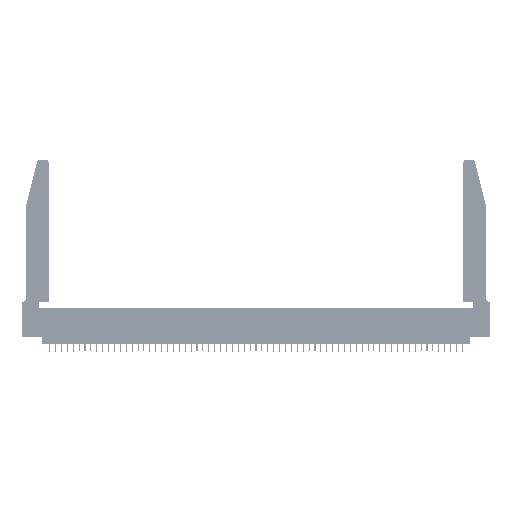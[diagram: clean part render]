
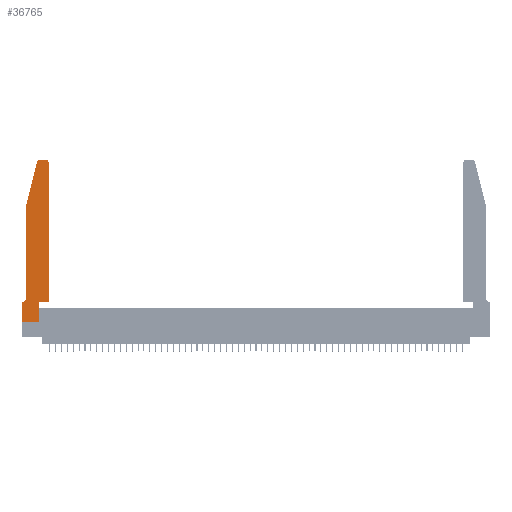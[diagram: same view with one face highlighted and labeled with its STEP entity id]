
A CAD part, top view. The second image highlights one B-rep face of the part: STEP entity #36765.
In plain terms, the highlighted planar face has unit normal (0, 0, 1).
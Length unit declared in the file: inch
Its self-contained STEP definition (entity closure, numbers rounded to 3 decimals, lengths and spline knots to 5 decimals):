
#133 = DIRECTION ( 'NONE',  ( -0.239, -0.971, 0. ) ) ;
#242 = VERTEX_POINT ( 'NONE', #3812 ) ;
#256 = CARTESIAN_POINT ( 'NONE',  ( 0.4205, 2.72, 0.37 ) ) ;
#416 = CARTESIAN_POINT ( 'NONE',  ( 0.0055, 0.42, 0.37 ) ) ;
#636 = DIRECTION ( 'NONE',  ( 0., 1., 0. ) ) ;
#1036 = CARTESIAN_POINT ( 'NONE',  ( 0.4505, 2.72, 0.37 ) ) ;
#1642 = VERTEX_POINT ( 'NONE', #56028 ) ;
#1770 = DIRECTION ( 'NONE',  ( 0., -1., 0. ) ) ;
#2079 = CARTESIAN_POINT ( 'NONE',  ( 0.2865, 0.35, 0.37 ) ) ;
#3624 = DIRECTION ( 'NONE',  ( 0., 0., -1. ) ) ;
#3812 = CARTESIAN_POINT ( 'NONE',  ( 0.0755, 0.42, 0.37 ) ) ;
#4233 = LINE ( 'NONE', #22372, #9941 ) ;
#4874 = EDGE_CURVE ( 'NONE', #10072, #18969, #46197, .T. ) ;
#4954 = LINE ( 'NONE', #40005, #13752 ) ;
#6051 = CARTESIAN_POINT ( 'NONE',  ( 0., 0.35, 0.37 ) ) ;
#8897 = DIRECTION ( 'NONE',  ( 1., 0., 0. ) ) ;
#8932 = EDGE_CURVE ( 'NONE', #41406, #28362, #38608, .T. ) ;
#9508 = CARTESIAN_POINT ( 'NONE',  ( 0.4205, 2.75, 0.37 ) ) ;
#9941 = VECTOR ( 'NONE', #21232, 39.37008 ) ;
#10072 = VERTEX_POINT ( 'NONE', #12974 ) ;
#10731 = VERTEX_POINT ( 'NONE', #45326 ) ;
#11606 = AXIS2_PLACEMENT_3D ( 'NONE', #15810, #56306, #50840 ) ;
#11866 = VERTEX_POINT ( 'NONE', #34751 ) ;
#12131 = AXIS2_PLACEMENT_3D ( 'NONE', #416, #3624, #21180 ) ;
#12811 = CARTESIAN_POINT ( 'NONE',  ( 0.0755, 2., 0.37 ) ) ;
#12974 = CARTESIAN_POINT ( 'NONE',  ( 0.284, 2.75, 0.37 ) ) ;
#13752 = VECTOR ( 'NONE', #636, 39.37008 ) ;
#14087 = EDGE_CURVE ( 'NONE', #1642, #19482, #4233, .T. ) ;
#14228 = LINE ( 'NONE', #48415, #37385 ) ;
#14549 = DIRECTION ( 'NONE',  ( 1., 0., 0. ) ) ;
#14752 = DIRECTION ( 'NONE',  ( 1., 0., 0. ) ) ;
#15810 = CARTESIAN_POINT ( 'NONE',  ( 0., 0.35, 0.37 ) ) ;
#15843 = EDGE_CURVE ( 'NONE', #18969, #26287, #36752, .T. ) ;
#15962 = ORIENTED_EDGE ( 'NONE', *, *, #15843, .T. ) ;
#17967 = DIRECTION ( 'NONE',  ( 1., 0., 0. ) ) ;
#18969 = VERTEX_POINT ( 'NONE', #40015 ) ;
#19440 = VERTEX_POINT ( 'NONE', #9508 ) ;
#19482 = VERTEX_POINT ( 'NONE', #6051 ) ;
#19561 = FACE_OUTER_BOUND ( 'NONE', #33764, .T. ) ;
#21128 = DIRECTION ( 'NONE',  ( 0., 1., 0. ) ) ;
#21180 = DIRECTION ( 'NONE',  ( -1., 0., 0. ) ) ;
#21232 = DIRECTION ( 'NONE',  ( -1., 0., 0. ) ) ;
#21454 = AXIS2_PLACEMENT_3D ( 'NONE', #40386, #35789, #14549 ) ;
#21631 = VERTEX_POINT ( 'NONE', #1036 ) ;
#22372 = CARTESIAN_POINT ( 'NONE',  ( 0.0755, 0.35, 0.37 ) ) ;
#23289 = EDGE_CURVE ( 'NONE', #11866, #41406, #14228, .T. ) ;
#23376 = VECTOR ( 'NONE', #28044, 39.37008 ) ;
#23929 = LINE ( 'NONE', #33097, #39742 ) ;
#25244 = EDGE_CURVE ( 'NONE', #28362, #10731, #36829, .T. ) ;
#26287 = VERTEX_POINT ( 'NONE', #52406 ) ;
#27281 = DIRECTION ( 'NONE',  ( 0., 0., 1. ) ) ;
#27922 = ORIENTED_EDGE ( 'NONE', *, *, #47736, .T. ) ;
#28044 = DIRECTION ( 'NONE',  ( -1., 0., 0. ) ) ;
#28362 = VERTEX_POINT ( 'NONE', #2079 ) ;
#29214 = ORIENTED_EDGE ( 'NONE', *, *, #42809, .T. ) ;
#30078 = ORIENTED_EDGE ( 'NONE', *, *, #39623, .T. ) ;
#30539 = EDGE_CURVE ( 'NONE', #242, #1642, #53443, .T. ) ;
#30883 = ORIENTED_EDGE ( 'NONE', *, *, #32994, .T. ) ;
#31133 = CARTESIAN_POINT ( 'NONE',  ( 0., 0., 0.37 ) ) ;
#32994 = EDGE_CURVE ( 'NONE', #26287, #242, #23929, .T. ) ;
#33097 = CARTESIAN_POINT ( 'NONE',  ( 0.0755, 2., 0.37 ) ) ;
#33535 = VECTOR ( 'NONE', #21128, 39.37008 ) ;
#33764 = EDGE_LOOP ( 'NONE', ( #27922, #39253, #15962, #30883, #53707, #35197, #30078, #39022, #38485, #50624, #29214, #34914 ) ) ;
#33943 = VECTOR ( 'NONE', #133, 39.37008 ) ;
#34751 = CARTESIAN_POINT ( 'NONE',  ( 0., 0., 0.37 ) ) ;
#34914 = ORIENTED_EDGE ( 'NONE', *, *, #43722, .T. ) ;
#35197 = ORIENTED_EDGE ( 'NONE', *, *, #14087, .T. ) ;
#35789 = DIRECTION ( 'NONE',  ( 0., 0., 1. ) ) ;
#36752 = LINE ( 'NONE', #12811, #33943 ) ;
#36765 = ADVANCED_FACE ( 'NONE', ( #19561 ), #42214, .T. ) ;
#36829 = LINE ( 'NONE', #37955, #45639 ) ;
#37385 = VECTOR ( 'NONE', #17967, 39.37008 ) ;
#37955 = CARTESIAN_POINT ( 'NONE',  ( 0.4505, 0.35, 0.37 ) ) ;
#38485 = ORIENTED_EDGE ( 'NONE', *, *, #8932, .T. ) ;
#38608 = LINE ( 'NONE', #46959, #33535 ) ;
#39022 = ORIENTED_EDGE ( 'NONE', *, *, #23289, .T. ) ;
#39253 = ORIENTED_EDGE ( 'NONE', *, *, #4874, .T. ) ;
#39520 = AXIS2_PLACEMENT_3D ( 'NONE', #256, #27281, #8897 ) ;
#39623 = EDGE_CURVE ( 'NONE', #19482, #11866, #39985, .T. ) ;
#39742 = VECTOR ( 'NONE', #50316, 39.37008 ) ;
#39985 = LINE ( 'NONE', #31133, #49295 ) ;
#40005 = CARTESIAN_POINT ( 'NONE',  ( 0.4505, 0.35, 0.37 ) ) ;
#40015 = CARTESIAN_POINT ( 'NONE',  ( 0.25487, 2.72718, 0.37 ) ) ;
#40386 = CARTESIAN_POINT ( 'NONE',  ( 0.284, 2.72, 0.37 ) ) ;
#41406 = VERTEX_POINT ( 'NONE', #54318 ) ;
#41799 = CARTESIAN_POINT ( 'NONE',  ( 0.2605, 2.75, 0.37 ) ) ;
#42214 = PLANE ( 'NONE',  #11606 ) ;
#42809 = EDGE_CURVE ( 'NONE', #10731, #21631, #4954, .T. ) ;
#43722 = EDGE_CURVE ( 'NONE', #21631, #19440, #49629, .T. ) ;
#45326 = CARTESIAN_POINT ( 'NONE',  ( 0.4505, 0.35, 0.37 ) ) ;
#45639 = VECTOR ( 'NONE', #14752, 39.37008 ) ;
#45839 = LINE ( 'NONE', #41799, #23376 ) ;
#46197 = CIRCLE ( 'NONE', #21454, 0.03 ) ;
#46959 = CARTESIAN_POINT ( 'NONE',  ( 0.2865, 0.35, 0.37 ) ) ;
#47736 = EDGE_CURVE ( 'NONE', #19440, #10072, #45839, .T. ) ;
#48415 = CARTESIAN_POINT ( 'NONE',  ( 0., 0., 0.37 ) ) ;
#49295 = VECTOR ( 'NONE', #1770, 39.37008 ) ;
#49629 = CIRCLE ( 'NONE', #39520, 0.03 ) ;
#50316 = DIRECTION ( 'NONE',  ( 0., -1., 0. ) ) ;
#50624 = ORIENTED_EDGE ( 'NONE', *, *, #25244, .T. ) ;
#50840 = DIRECTION ( 'NONE',  ( 1., 0., 0. ) ) ;
#52406 = CARTESIAN_POINT ( 'NONE',  ( 0.0755, 2., 0.37 ) ) ;
#53443 = CIRCLE ( 'NONE', #12131, 0.07 ) ;
#53707 = ORIENTED_EDGE ( 'NONE', *, *, #30539, .T. ) ;
#54318 = CARTESIAN_POINT ( 'NONE',  ( 0.2865, 0., 0.37 ) ) ;
#56028 = CARTESIAN_POINT ( 'NONE',  ( 0.0055, 0.35, 0.37 ) ) ;
#56306 = DIRECTION ( 'NONE',  ( 0., 0., 1. ) ) ;
